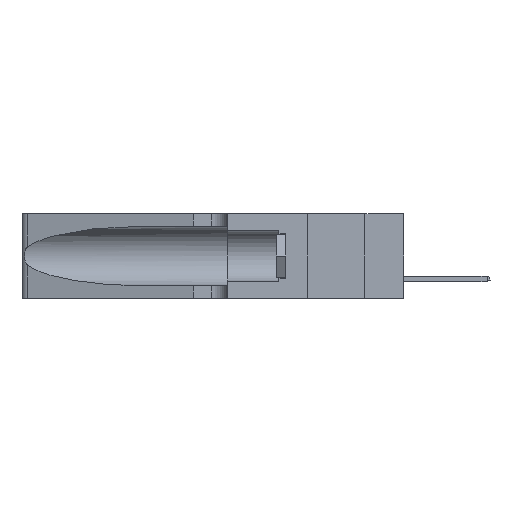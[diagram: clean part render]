
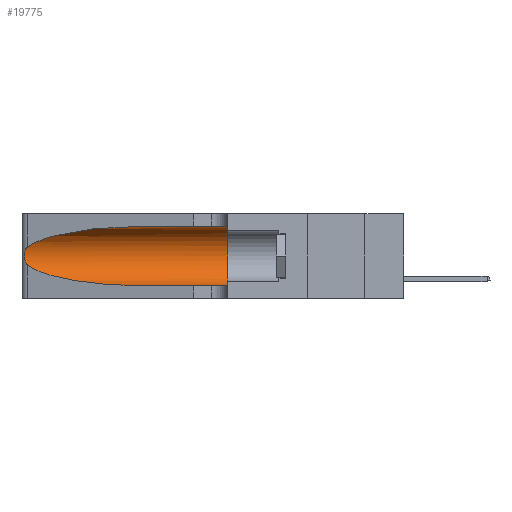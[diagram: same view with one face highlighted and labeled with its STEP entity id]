
A CAD part, left-side view. The second image highlights one B-rep face of the part: STEP entity #19775.
In plain terms, the highlighted cylindrical face has radius 3.308 mm (diameter 6.617 mm), a partial arc.
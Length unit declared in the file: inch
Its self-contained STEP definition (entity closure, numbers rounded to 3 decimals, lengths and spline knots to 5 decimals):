
#97 = CARTESIAN_POINT ( 'NONE',  ( 0.26018, 1.23835, 0.19895 ) ) ;
#589 = EDGE_CURVE ( 'NONE', #1624, #9876, #8478, .T. ) ;
#1141 = ORIENTED_EDGE ( 'NONE', *, *, #14382, .F. ) ;
#1223 = CARTESIAN_POINT ( 'NONE',  ( 0.25487, 1.22718, 0.14631 ) ) ;
#1265 = VERTEX_POINT ( 'NONE', #9113 ) ;
#1624 = VERTEX_POINT ( 'NONE', #20230 ) ;
#1697 = CARTESIAN_POINT ( 'NONE',  ( 0.26075, 1.23896, 0.178 ) ) ;
#1897 = CARTESIAN_POINT ( 'NONE',  ( 0.25789, 1.23486, 0.15765 ) ) ;
#2051 = CARTESIAN_POINT ( 'NONE',  ( 0.2373, 1.15595, 0.08982 ) ) ;
#2528 = CARTESIAN_POINT ( 'NONE',  ( 0.1305, 1.61858, 0.185 ) ) ;
#2760 = DIRECTION ( 'NONE',  ( 0., 0., 1. ) ) ;
#3192 = ORIENTED_EDGE ( 'NONE', *, *, #11008, .T. ) ;
#3535 = CARTESIAN_POINT ( 'NONE',  ( 0.25487, 1.22718, 0.22369 ) ) ;
#3685 = CARTESIAN_POINT ( 'NONE',  ( 0.1305, 0.35, 0.05475 ) ) ;
#3910 = VECTOR ( 'NONE', #14053, 39.37008 ) ;
#4165 = LINE ( 'NONE', #20283, #3910 ) ;
#4313 = VERTEX_POINT ( 'NONE', #3685 ) ;
#5693 = FACE_OUTER_BOUND ( 'NONE', #17371, .T. ) ;
#5910 = CARTESIAN_POINT ( 'NONE',  ( 0.1305, 0.35, 0.31525 ) ) ;
#6264 = CIRCLE ( 'NONE', #20036, 0.13025 ) ;
#6426 = CARTESIAN_POINT ( 'NONE',  ( 0.25856, 1.23593, 0.16098 ) ) ;
#6520 = CARTESIAN_POINT ( 'NONE',  ( 0.1305, 0.72297, 0.05475 ) ) ;
#6684 =( BOUNDED_CURVE ( )  B_SPLINE_CURVE ( 3, ( #11258, #2051, #14426, #6520 ),
 .UNSPECIFIED., .F., .T. ) 
 B_SPLINE_CURVE_WITH_KNOTS ( ( 4, 4 ),
 ( 3.44316, 4.71239 ),
 .UNSPECIFIED. ) 
 CURVE ( )  GEOMETRIC_REPRESENTATION_ITEM ( )  RATIONAL_B_SPLINE_CURVE ( ( 1., 0.87, 0.87, 1. ) ) 
 REPRESENTATION_ITEM ( '' )  );
#7200 = DIRECTION ( 'NONE',  ( 0., -1., 0. ) ) ;
#7720 = CARTESIAN_POINT ( 'NONE',  ( 0.1305, 1.61858, 0.31525 ) ) ;
#7849 =( BOUNDED_CURVE ( )  B_SPLINE_CURVE ( 3, ( #14348, #12911, #11186, #3535 ),
 .UNSPECIFIED., .F., .F. ) 
 B_SPLINE_CURVE_WITH_KNOTS ( ( 4, 4 ),
 ( 1.5708, 2.84003 ),
 .UNSPECIFIED. ) 
 CURVE ( )  GEOMETRIC_REPRESENTATION_ITEM ( )  RATIONAL_B_SPLINE_CURVE ( ( 1., 0.87, 0.87, 1. ) ) 
 REPRESENTATION_ITEM ( '' )  );
#8030 = CARTESIAN_POINT ( 'NONE',  ( 0.25555, 1.22993, 0.14849 ) ) ;
#8152 = VECTOR ( 'NONE', #14557, 39.37008 ) ;
#8478 = B_SPLINE_CURVE_WITH_KNOTS ( 'NONE', 3,
 ( #11240, #15971, #9734, #15764, #17347, #97, #11307, #1697, #12698, #6426, #1897, #12902, #8030, #18965 ),
 .UNSPECIFIED., .F., .F.,
 ( 4, 2, 2, 2, 2, 2, 4 ),
 ( 0., 0.00027, 0.00053, 0.00107, 0.0016, 0.00187, 0.00214 ),
 .UNSPECIFIED. ) ;
#9029 = ORIENTED_EDGE ( 'NONE', *, *, #10914, .F. ) ;
#9113 = CARTESIAN_POINT ( 'NONE',  ( 0.1305, 0.72297, 0.31525 ) ) ;
#9146 = DIRECTION ( 'NONE',  ( 0., 1., 0. ) ) ;
#9228 = ORIENTED_EDGE ( 'NONE', *, *, #589, .T. ) ;
#9573 = AXIS2_PLACEMENT_3D ( 'NONE', #2528, #7200, #11876 ) ;
#9734 = CARTESIAN_POINT ( 'NONE',  ( 0.25639, 1.23184, 0.21858 ) ) ;
#9876 = VERTEX_POINT ( 'NONE', #1223 ) ;
#10852 = VERTEX_POINT ( 'NONE', #14505 ) ;
#10866 = LINE ( 'NONE', #7720, #8152 ) ;
#10914 = EDGE_CURVE ( 'NONE', #1265, #19197, #10866, .T. ) ;
#11008 = EDGE_CURVE ( 'NONE', #9876, #10852, #6684, .T. ) ;
#11186 = CARTESIAN_POINT ( 'NONE',  ( 0.2373, 1.15595, 0.28018 ) ) ;
#11240 = CARTESIAN_POINT ( 'NONE',  ( 0.25487, 1.22718, 0.22369 ) ) ;
#11258 = CARTESIAN_POINT ( 'NONE',  ( 0.25487, 1.22718, 0.14631 ) ) ;
#11307 = CARTESIAN_POINT ( 'NONE',  ( 0.26075, 1.23896, 0.19203 ) ) ;
#11396 = EDGE_CURVE ( 'NONE', #10852, #4313, #4165, .T. ) ;
#11876 = DIRECTION ( 'NONE',  ( 0., 0., -1. ) ) ;
#12698 = CARTESIAN_POINT ( 'NONE',  ( 0.26017, 1.23833, 0.17102 ) ) ;
#12902 = CARTESIAN_POINT ( 'NONE',  ( 0.25639, 1.23186, 0.15144 ) ) ;
#12911 = CARTESIAN_POINT ( 'NONE',  ( 0.18966, 0.96281, 0.31525 ) ) ;
#14048 = CYLINDRICAL_SURFACE ( 'NONE', #9573, 0.13025 ) ;
#14053 = DIRECTION ( 'NONE',  ( 0., -1., 0. ) ) ;
#14348 = CARTESIAN_POINT ( 'NONE',  ( 0.1305, 0.72297, 0.31525 ) ) ;
#14382 = EDGE_CURVE ( 'NONE', #19197, #4313, #6264, .T. ) ;
#14426 = CARTESIAN_POINT ( 'NONE',  ( 0.18966, 0.96281, 0.05475 ) ) ;
#14505 = CARTESIAN_POINT ( 'NONE',  ( 0.1305, 0.72297, 0.05475 ) ) ;
#14557 = DIRECTION ( 'NONE',  ( 0., -1., 0. ) ) ;
#15420 = ORIENTED_EDGE ( 'NONE', *, *, #11396, .T. ) ;
#15764 = CARTESIAN_POINT ( 'NONE',  ( 0.25787, 1.23484, 0.2124 ) ) ;
#15971 = CARTESIAN_POINT ( 'NONE',  ( 0.25555, 1.22994, 0.2215 ) ) ;
#16870 = ORIENTED_EDGE ( 'NONE', *, *, #19501, .T. ) ;
#17347 = CARTESIAN_POINT ( 'NONE',  ( 0.25854, 1.2359, 0.20912 ) ) ;
#17371 = EDGE_LOOP ( 'NONE', ( #16870, #9228, #3192, #15420, #1141, #9029 ) ) ;
#18586 = CARTESIAN_POINT ( 'NONE',  ( 0.1305, 0.35, 0.185 ) ) ;
#18965 = CARTESIAN_POINT ( 'NONE',  ( 0.25487, 1.22718, 0.14631 ) ) ;
#19197 = VERTEX_POINT ( 'NONE', #5910 ) ;
#19501 = EDGE_CURVE ( 'NONE', #1265, #1624, #7849, .T. ) ;
#19775 = ADVANCED_FACE ( 'NONE', ( #5693 ), #14048, .F. ) ;
#20036 = AXIS2_PLACEMENT_3D ( 'NONE', #18586, #9146, #2760 ) ;
#20230 = CARTESIAN_POINT ( 'NONE',  ( 0.25487, 1.22718, 0.22369 ) ) ;
#20283 = CARTESIAN_POINT ( 'NONE',  ( 0.1305, 1.61858, 0.05475 ) ) ;
